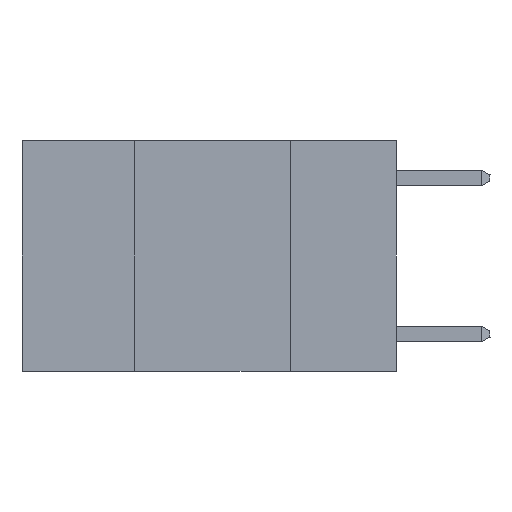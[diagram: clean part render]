
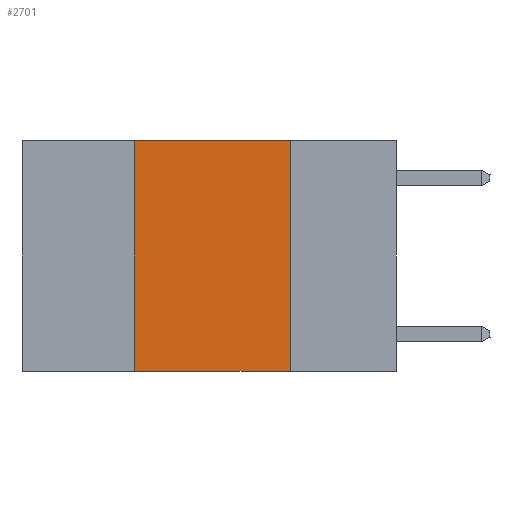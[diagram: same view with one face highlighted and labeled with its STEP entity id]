
A CAD part, left-side view. The second image highlights one B-rep face of the part: STEP entity #2701.
In plain terms, the highlighted planar face has unit normal (-1, 0, 0).
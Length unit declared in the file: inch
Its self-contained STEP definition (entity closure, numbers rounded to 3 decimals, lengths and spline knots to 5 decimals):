
#513 = ORIENTED_EDGE ( 'NONE', *, *, #5462, .F. ) ;
#1015 = LINE ( 'NONE', #1673, #2962 ) ;
#1016 = VERTEX_POINT ( 'NONE', #7705 ) ;
#1052 = DIRECTION ( 'NONE',  ( 0., -1., 0. ) ) ;
#1445 = EDGE_LOOP ( 'NONE', ( #2791, #9323, #513, #5506 ) ) ;
#1673 = CARTESIAN_POINT ( 'NONE',  ( 0., 0.6, 0. ) ) ;
#1707 = DIRECTION ( 'NONE',  ( 0., 0., 1. ) ) ;
#2111 = DIRECTION ( 'NONE',  ( 0., 0., -1. ) ) ;
#2140 = CARTESIAN_POINT ( 'NONE',  ( 0., 0.17, 0. ) ) ;
#2454 = PLANE ( 'NONE',  #10681 ) ;
#2526 = EDGE_CURVE ( 'NONE', #3479, #1016, #6750, .T. ) ;
#2701 = ADVANCED_FACE ( 'NONE', ( #9675 ), #2454, .F. ) ;
#2791 = ORIENTED_EDGE ( 'NONE', *, *, #2526, .F. ) ;
#2962 = VECTOR ( 'NONE', #6386, 39.37008 ) ;
#3466 = DIRECTION ( 'NONE',  ( 0., 0., -1. ) ) ;
#3479 = VERTEX_POINT ( 'NONE', #2140 ) ;
#3901 = VERTEX_POINT ( 'NONE', #7568 ) ;
#3953 = CARTESIAN_POINT ( 'NONE',  ( 0., 0.17, 0. ) ) ;
#5462 = EDGE_CURVE ( 'NONE', #6564, #3901, #8125, .T. ) ;
#5506 = ORIENTED_EDGE ( 'NONE', *, *, #5561, .T. ) ;
#5561 = EDGE_CURVE ( 'NONE', #6564, #1016, #6302, .T. ) ;
#6302 = LINE ( 'NONE', #9805, #9044 ) ;
#6359 = CARTESIAN_POINT ( 'NONE',  ( 0., 0.42, 0. ) ) ;
#6386 = DIRECTION ( 'NONE',  ( 0., -1., 0. ) ) ;
#6564 = VERTEX_POINT ( 'NONE', #11317 ) ;
#6750 = LINE ( 'NONE', #3953, #11052 ) ;
#7015 = CARTESIAN_POINT ( 'NONE',  ( 0., 0.6, 0. ) ) ;
#7568 = CARTESIAN_POINT ( 'NONE',  ( 0., 0.42, 0. ) ) ;
#7705 = CARTESIAN_POINT ( 'NONE',  ( 0., 0.17, -0.37 ) ) ;
#7777 = DIRECTION ( 'NONE',  ( 1., 0., 0. ) ) ;
#7931 = VECTOR ( 'NONE', #1707, 39.37008 ) ;
#8125 = LINE ( 'NONE', #6359, #7931 ) ;
#9044 = VECTOR ( 'NONE', #1052, 39.37008 ) ;
#9323 = ORIENTED_EDGE ( 'NONE', *, *, #10239, .F. ) ;
#9675 = FACE_OUTER_BOUND ( 'NONE', #1445, .T. ) ;
#9805 = CARTESIAN_POINT ( 'NONE',  ( 0., 0.6, -0.37 ) ) ;
#10239 = EDGE_CURVE ( 'NONE', #3901, #3479, #1015, .T. ) ;
#10681 = AXIS2_PLACEMENT_3D ( 'NONE', #7015, #7777, #3466 ) ;
#11052 = VECTOR ( 'NONE', #2111, 39.37008 ) ;
#11317 = CARTESIAN_POINT ( 'NONE',  ( 0., 0.42, -0.37 ) ) ;
